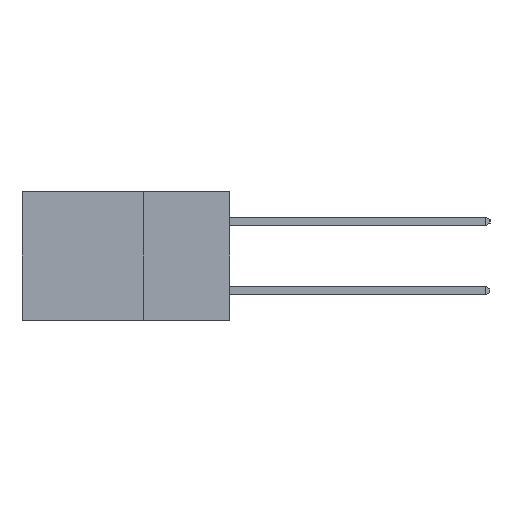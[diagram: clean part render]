
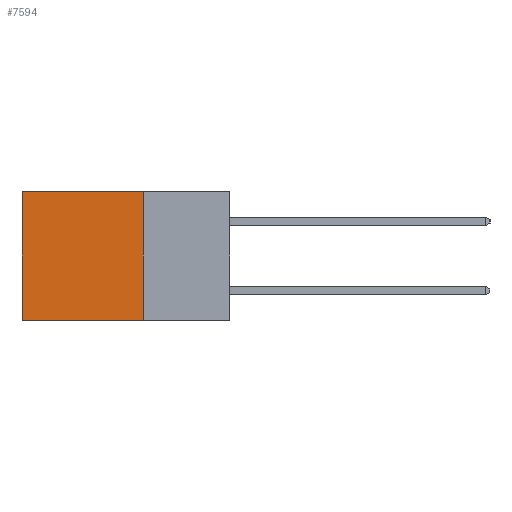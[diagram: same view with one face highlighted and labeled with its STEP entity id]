
A CAD part, left-side view. The second image highlights one B-rep face of the part: STEP entity #7594.
In plain terms, the highlighted planar face has unit normal (-1, 0, 0).
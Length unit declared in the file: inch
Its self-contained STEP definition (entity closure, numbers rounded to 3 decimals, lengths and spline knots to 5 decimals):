
#695 = DIRECTION ( 'NONE',  ( 0., 1., 0. ) ) ;
#1210 = VERTEX_POINT ( 'NONE', #10822 ) ;
#1424 = VERTEX_POINT ( 'NONE', #2384 ) ;
#2045 = CARTESIAN_POINT ( 'NONE',  ( 0.298, 0.25, -0.37 ) ) ;
#2130 = FACE_OUTER_BOUND ( 'NONE', #2881, .T. ) ;
#2384 = CARTESIAN_POINT ( 'NONE',  ( 0.298, 0.25, -0.37 ) ) ;
#2819 = CARTESIAN_POINT ( 'NONE',  ( 0.298, 0.6, 0. ) ) ;
#2881 = EDGE_LOOP ( 'NONE', ( #13575, #3466, #8145, #6159 ) ) ;
#3113 = CARTESIAN_POINT ( 'NONE',  ( 0.298, 0.25, 0. ) ) ;
#3198 = VECTOR ( 'NONE', #13816, 39.37008 ) ;
#3466 = ORIENTED_EDGE ( 'NONE', *, *, #8166, .F. ) ;
#4243 = DIRECTION ( 'NONE',  ( 0., 0., -1. ) ) ;
#4392 = LINE ( 'NONE', #3113, #12375 ) ;
#4506 = DIRECTION ( 'NONE',  ( 0., 0., -1. ) ) ;
#6159 = ORIENTED_EDGE ( 'NONE', *, *, #7526, .T. ) ;
#6404 = LINE ( 'NONE', #13766, #3198 ) ;
#6472 = EDGE_CURVE ( 'NONE', #11848, #1210, #11681, .T. ) ;
#7071 = AXIS2_PLACEMENT_3D ( 'NONE', #11715, #11673, #10999 ) ;
#7526 = EDGE_CURVE ( 'NONE', #11433, #11848, #6404, .T. ) ;
#7557 = CARTESIAN_POINT ( 'NONE',  ( 0.298, 0.6, 0. ) ) ;
#7594 = ADVANCED_FACE ( 'NONE', ( #2130 ), #10907, .F. ) ;
#7731 = CARTESIAN_POINT ( 'NONE',  ( 0.298, 0.25, 0. ) ) ;
#8145 = ORIENTED_EDGE ( 'NONE', *, *, #13047, .F. ) ;
#8166 = EDGE_CURVE ( 'NONE', #1424, #1210, #13209, .T. ) ;
#8213 = VECTOR ( 'NONE', #695, 39.37008 ) ;
#8834 = VECTOR ( 'NONE', #4506, 39.37008 ) ;
#10822 = CARTESIAN_POINT ( 'NONE',  ( 0.298, 0.6, -0.37 ) ) ;
#10907 = PLANE ( 'NONE',  #7071 ) ;
#10999 = DIRECTION ( 'NONE',  ( 0., 0., -1. ) ) ;
#11433 = VERTEX_POINT ( 'NONE', #7731 ) ;
#11673 = DIRECTION ( 'NONE',  ( 1., 0., 0. ) ) ;
#11681 = LINE ( 'NONE', #2819, #8834 ) ;
#11715 = CARTESIAN_POINT ( 'NONE',  ( 0.298, 0.25, 0. ) ) ;
#11848 = VERTEX_POINT ( 'NONE', #7557 ) ;
#12375 = VECTOR ( 'NONE', #4243, 39.37008 ) ;
#13047 = EDGE_CURVE ( 'NONE', #11433, #1424, #4392, .T. ) ;
#13209 = LINE ( 'NONE', #2045, #8213 ) ;
#13575 = ORIENTED_EDGE ( 'NONE', *, *, #6472, .T. ) ;
#13766 = CARTESIAN_POINT ( 'NONE',  ( 0.298, 0.25, 0. ) ) ;
#13816 = DIRECTION ( 'NONE',  ( 0., 1., 0. ) ) ;
